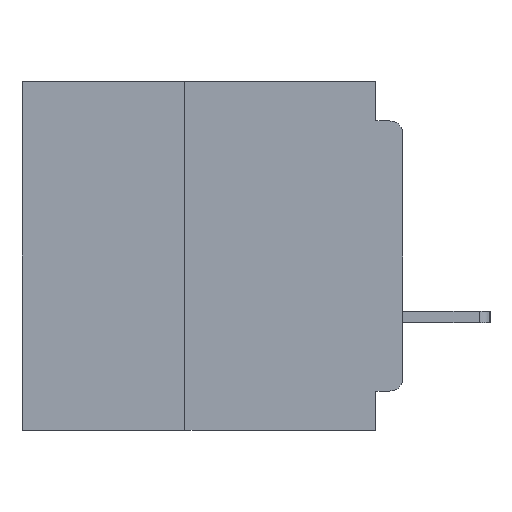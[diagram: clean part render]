
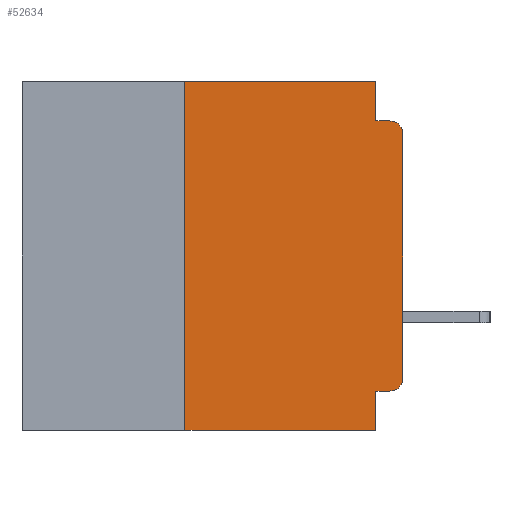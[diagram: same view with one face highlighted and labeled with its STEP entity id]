
A CAD part, left-side view. The second image highlights one B-rep face of the part: STEP entity #52634.
In plain terms, the highlighted planar face has unit normal (-1, 0, 0).
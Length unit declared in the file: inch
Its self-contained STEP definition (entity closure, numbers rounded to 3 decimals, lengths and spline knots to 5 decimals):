
#559 = VERTEX_POINT ( 'NONE', #38914 ) ;
#913 = EDGE_CURVE ( 'NONE', #25208, #47881, #17369, .T. ) ;
#1014 = CIRCLE ( 'NONE', #46521, 0.015 ) ;
#1490 = DIRECTION ( 'NONE',  ( 0., 0., -1. ) ) ;
#2400 = CIRCLE ( 'NONE', #23899, 0.015 ) ;
#3112 = CARTESIAN_POINT ( 'NONE',  ( 0., 0.25, -0.4 ) ) ;
#4417 = EDGE_CURVE ( 'NONE', #37762, #25208, #20871, .T. ) ;
#4833 = VECTOR ( 'NONE', #29496, 39.37008 ) ;
#5560 = CARTESIAN_POINT ( 'NONE',  ( 0., 0., 0. ) ) ;
#5612 = CARTESIAN_POINT ( 'NONE',  ( 0., 0.437, 0. ) ) ;
#5628 = VERTEX_POINT ( 'NONE', #35765 ) ;
#6552 = CARTESIAN_POINT ( 'NONE',  ( 0., 0., -0.355 ) ) ;
#6712 = CARTESIAN_POINT ( 'NONE',  ( 0., 0.25, -0.4 ) ) ;
#7008 = EDGE_CURVE ( 'NONE', #44448, #47881, #35043, .T. ) ;
#9782 = DIRECTION ( 'NONE',  ( 0., 0., -1. ) ) ;
#10319 = ORIENTED_EDGE ( 'NONE', *, *, #42056, .T. ) ;
#10471 = DIRECTION ( 'NONE',  ( 0., -1., 0. ) ) ;
#10649 = CARTESIAN_POINT ( 'NONE',  ( 0., 0.437, 0. ) ) ;
#10852 = FACE_OUTER_BOUND ( 'NONE', #15429, .T. ) ;
#11823 = ORIENTED_EDGE ( 'NONE', *, *, #15976, .F. ) ;
#11897 = LINE ( 'NONE', #32696, #32630 ) ;
#12718 = CARTESIAN_POINT ( 'NONE',  ( 0., 0.031, -0.4 ) ) ;
#13040 = VECTOR ( 'NONE', #39879, 39.37008 ) ;
#13103 = CARTESIAN_POINT ( 'NONE',  ( 0., 0.031, -0.045 ) ) ;
#13489 = AXIS2_PLACEMENT_3D ( 'NONE', #5612, #34580, #9782 ) ;
#14341 = ORIENTED_EDGE ( 'NONE', *, *, #16452, .F. ) ;
#15429 = EDGE_LOOP ( 'NONE', ( #39669, #10319, #14341, #11823, #47696, #18199, #34437, #21840, #43206, #37585 ) ) ;
#15976 = EDGE_CURVE ( 'NONE', #21538, #23458, #26853, .T. ) ;
#15991 = DIRECTION ( 'NONE',  ( -1., 0., 0. ) ) ;
#16061 = DIRECTION ( 'NONE',  ( 0., -1., 0. ) ) ;
#16452 = EDGE_CURVE ( 'NONE', #23458, #41551, #11897, .T. ) ;
#17369 = LINE ( 'NONE', #12718, #36756 ) ;
#18199 = ORIENTED_EDGE ( 'NONE', *, *, #28735, .F. ) ;
#18553 = LINE ( 'NONE', #5560, #50217 ) ;
#19046 = DIRECTION ( 'NONE',  ( 0., 1., 0. ) ) ;
#19167 = LINE ( 'NONE', #3112, #52160 ) ;
#19337 = EDGE_CURVE ( 'NONE', #5628, #559, #18553, .T. ) ;
#20871 = LINE ( 'NONE', #6552, #30603 ) ;
#21416 = CARTESIAN_POINT ( 'NONE',  ( 0., 0.031, -0.355 ) ) ;
#21538 = VERTEX_POINT ( 'NONE', #33710 ) ;
#21840 = ORIENTED_EDGE ( 'NONE', *, *, #913, .F. ) ;
#23458 = VERTEX_POINT ( 'NONE', #13103 ) ;
#23899 = AXIS2_PLACEMENT_3D ( 'NONE', #51049, #26271, #1490 ) ;
#25208 = VERTEX_POINT ( 'NONE', #21416 ) ;
#26189 = DIRECTION ( 'NONE',  ( 0., 0., 1. ) ) ;
#26271 = DIRECTION ( 'NONE',  ( -1., 0., 0. ) ) ;
#26853 = LINE ( 'NONE', #50083, #4833 ) ;
#28735 = EDGE_CURVE ( 'NONE', #44448, #40951, #19167, .T. ) ;
#29434 = CARTESIAN_POINT ( 'NONE',  ( 0., 0.015, -0.045 ) ) ;
#29496 = DIRECTION ( 'NONE',  ( 0., 0., -1. ) ) ;
#29817 = EDGE_CURVE ( 'NONE', #40951, #21538, #31975, .T. ) ;
#30544 = DIRECTION ( 'NONE',  ( 0., 0., -1. ) ) ;
#30603 = VECTOR ( 'NONE', #19046, 39.37008 ) ;
#30871 = EDGE_CURVE ( 'NONE', #37762, #5628, #2400, .T. ) ;
#31975 = LINE ( 'NONE', #10649, #52663 ) ;
#32630 = VECTOR ( 'NONE', #16061, 39.37008 ) ;
#32696 = CARTESIAN_POINT ( 'NONE',  ( 0., 0., -0.045 ) ) ;
#33475 = CARTESIAN_POINT ( 'NONE',  ( 0., 0.015, -0.355 ) ) ;
#33710 = CARTESIAN_POINT ( 'NONE',  ( 0., 0.031, 0. ) ) ;
#33841 = CARTESIAN_POINT ( 'NONE',  ( 0., 0.25, 0. ) ) ;
#34437 = ORIENTED_EDGE ( 'NONE', *, *, #7008, .T. ) ;
#34580 = DIRECTION ( 'NONE',  ( 1., 0., 0. ) ) ;
#35043 = LINE ( 'NONE', #52341, #13040 ) ;
#35765 = CARTESIAN_POINT ( 'NONE',  ( 0., 0., -0.34 ) ) ;
#36087 = DIRECTION ( 'NONE',  ( 0., 0., 1. ) ) ;
#36756 = VECTOR ( 'NONE', #30544, 39.37008 ) ;
#37585 = ORIENTED_EDGE ( 'NONE', *, *, #30871, .T. ) ;
#37762 = VERTEX_POINT ( 'NONE', #33475 ) ;
#38914 = CARTESIAN_POINT ( 'NONE',  ( 0., 0., -0.06 ) ) ;
#39669 = ORIENTED_EDGE ( 'NONE', *, *, #19337, .T. ) ;
#39879 = DIRECTION ( 'NONE',  ( 0., -1., 0. ) ) ;
#40754 = CARTESIAN_POINT ( 'NONE',  ( 0., 0.015, -0.06 ) ) ;
#40951 = VERTEX_POINT ( 'NONE', #33841 ) ;
#41551 = VERTEX_POINT ( 'NONE', #29434 ) ;
#42056 = EDGE_CURVE ( 'NONE', #559, #41551, #1014, .T. ) ;
#43206 = ORIENTED_EDGE ( 'NONE', *, *, #4417, .F. ) ;
#44448 = VERTEX_POINT ( 'NONE', #6712 ) ;
#44910 = DIRECTION ( 'NONE',  ( 0., 0., -1. ) ) ;
#46521 = AXIS2_PLACEMENT_3D ( 'NONE', #40754, #15991, #44910 ) ;
#47696 = ORIENTED_EDGE ( 'NONE', *, *, #29817, .F. ) ;
#47881 = VERTEX_POINT ( 'NONE', #51947 ) ;
#50083 = CARTESIAN_POINT ( 'NONE',  ( 0., 0.031, 0. ) ) ;
#50217 = VECTOR ( 'NONE', #26189, 39.37008 ) ;
#51016 = PLANE ( 'NONE',  #13489 ) ;
#51049 = CARTESIAN_POINT ( 'NONE',  ( 0., 0.015, -0.34 ) ) ;
#51947 = CARTESIAN_POINT ( 'NONE',  ( 0., 0.031, -0.4 ) ) ;
#52160 = VECTOR ( 'NONE', #36087, 39.37008 ) ;
#52341 = CARTESIAN_POINT ( 'NONE',  ( 0., 0.437, -0.4 ) ) ;
#52634 = ADVANCED_FACE ( 'NONE', ( #10852 ), #51016, .F. ) ;
#52663 = VECTOR ( 'NONE', #10471, 39.37008 ) ;
